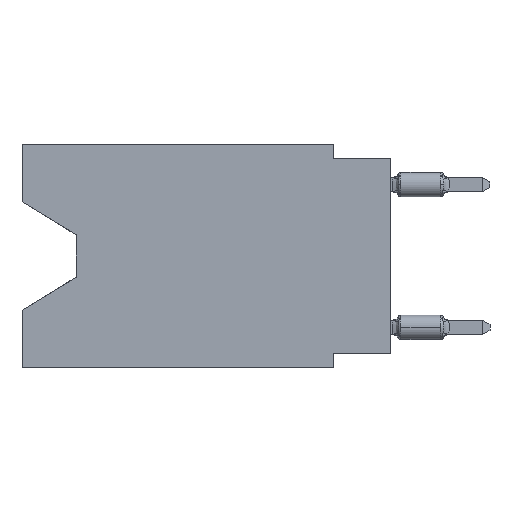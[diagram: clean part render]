
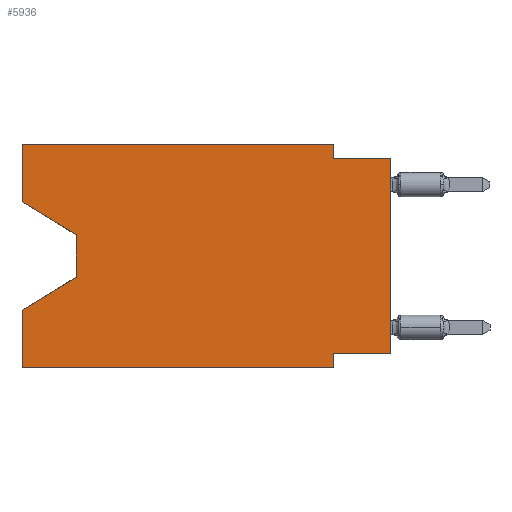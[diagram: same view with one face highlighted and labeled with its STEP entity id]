
A CAD part, left-side view. The second image highlights one B-rep face of the part: STEP entity #5936.
In plain terms, the highlighted planar face has unit normal (-1, 0, 0).
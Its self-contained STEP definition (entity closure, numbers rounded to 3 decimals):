
#179 = CARTESIAN_POINT ( 'NONE',  ( 0., 13.97, -4.013 ) ) ;
#182 = VERTEX_POINT ( 'NONE', #1026 ) ;
#193 = EDGE_CURVE ( 'NONE', #15948, #651, #8616, .T. ) ;
#277 = EDGE_CURVE ( 'NONE', #6766, #4289, #13559, .T. ) ;
#651 = VERTEX_POINT ( 'NONE', #14524 ) ;
#699 = DIRECTION ( 'NONE',  ( 0., 0., 1. ) ) ;
#1026 = CARTESIAN_POINT ( 'NONE',  ( 0., 13.97, -4.013 ) ) ;
#1091 = EDGE_CURVE ( 'NONE', #10111, #4216, #5982, .T. ) ;
#1182 = EDGE_CURVE ( 'NONE', #4814, #3480, #11240, .T. ) ;
#1298 = CARTESIAN_POINT ( 'NONE',  ( 0., 16.383, 0. ) ) ;
#1342 = EDGE_CURVE ( 'NONE', #4814, #182, #1703, .T. ) ;
#1429 = VECTOR ( 'NONE', #1827, 1000. ) ;
#1532 = VERTEX_POINT ( 'NONE', #7032 ) ;
#1703 = LINE ( 'NONE', #11560, #4851 ) ;
#1827 = DIRECTION ( 'NONE',  ( 0., -1., 0. ) ) ;
#2109 = ORIENTED_EDGE ( 'NONE', *, *, #11986, .F. ) ;
#2229 = LINE ( 'NONE', #15488, #12310 ) ;
#2294 = EDGE_CURVE ( 'NONE', #651, #9453, #3707, .T. ) ;
#2566 = ORIENTED_EDGE ( 'NONE', *, *, #15207, .F. ) ;
#2656 = LINE ( 'NONE', #12366, #3254 ) ;
#3180 = CARTESIAN_POINT ( 'NONE',  ( 0., 2.54, -9.906 ) ) ;
#3254 = VECTOR ( 'NONE', #5497, 1000. ) ;
#3269 = VECTOR ( 'NONE', #3675, 1000. ) ;
#3368 = CARTESIAN_POINT ( 'NONE',  ( 0., 0., -9.271 ) ) ;
#3475 = ORIENTED_EDGE ( 'NONE', *, *, #1182, .F. ) ;
#3480 = VERTEX_POINT ( 'NONE', #11234 ) ;
#3675 = DIRECTION ( 'NONE',  ( 0., -1., 0. ) ) ;
#3707 = LINE ( 'NONE', #13510, #9254 ) ;
#4113 = LINE ( 'NONE', #179, #4996 ) ;
#4216 = VERTEX_POINT ( 'NONE', #4569 ) ;
#4289 = VERTEX_POINT ( 'NONE', #7324 ) ;
#4407 = DIRECTION ( 'NONE',  ( 0., -1., 0. ) ) ;
#4450 = CARTESIAN_POINT ( 'NONE',  ( 0., 16.383, -9.906 ) ) ;
#4569 = CARTESIAN_POINT ( 'NONE',  ( 0., 16.383, -7.36 ) ) ;
#4804 = DIRECTION ( 'NONE',  ( 0., 0., -1. ) ) ;
#4814 = VERTEX_POINT ( 'NONE', #11020 ) ;
#4851 = VECTOR ( 'NONE', #7923, 1000. ) ;
#4869 = VECTOR ( 'NONE', #12549, 1000. ) ;
#4996 = VECTOR ( 'NONE', #9055, 1000. ) ;
#5497 = DIRECTION ( 'NONE',  ( 0., 0., 1. ) ) ;
#5936 = ADVANCED_FACE ( 'NONE', ( #15030 ), #10025, .F. ) ;
#5982 = LINE ( 'NONE', #12224, #12646 ) ;
#6018 = CARTESIAN_POINT ( 'NONE',  ( 0., 2.54, 0. ) ) ;
#6459 = ORIENTED_EDGE ( 'NONE', *, *, #1342, .T. ) ;
#6766 = VERTEX_POINT ( 'NONE', #13468 ) ;
#6854 = LINE ( 'NONE', #15508, #8143 ) ;
#7004 = ORIENTED_EDGE ( 'NONE', *, *, #11305, .T. ) ;
#7032 = CARTESIAN_POINT ( 'NONE',  ( 0., 0., -0.635 ) ) ;
#7307 = ORIENTED_EDGE ( 'NONE', *, *, #15469, .F. ) ;
#7324 = CARTESIAN_POINT ( 'NONE',  ( 0., 2.54, -0.635 ) ) ;
#7740 = CARTESIAN_POINT ( 'NONE',  ( 0., 13.97, -5.893 ) ) ;
#7923 = DIRECTION ( 'NONE',  ( 0., -0.855, -0.519 ) ) ;
#7995 = VECTOR ( 'NONE', #4804, 1000. ) ;
#8143 = VECTOR ( 'NONE', #4407, 1000. ) ;
#8616 = LINE ( 'NONE', #3368, #11880 ) ;
#8837 = AXIS2_PLACEMENT_3D ( 'NONE', #10179, #9858, #11068 ) ;
#9055 = DIRECTION ( 'NONE',  ( 0., 0., -1. ) ) ;
#9254 = VECTOR ( 'NONE', #15842, 1000. ) ;
#9453 = VERTEX_POINT ( 'NONE', #3180 ) ;
#9573 = ORIENTED_EDGE ( 'NONE', *, *, #11644, .T. ) ;
#9858 = DIRECTION ( 'NONE',  ( 1., 0., 0. ) ) ;
#10025 = PLANE ( 'NONE',  #8837 ) ;
#10029 = ORIENTED_EDGE ( 'NONE', *, *, #193, .F. ) ;
#10111 = VERTEX_POINT ( 'NONE', #7740 ) ;
#10179 = CARTESIAN_POINT ( 'NONE',  ( 0., 16.383, 0. ) ) ;
#10734 = DIRECTION ( 'NONE',  ( 0., 1., 0. ) ) ;
#10851 = DIRECTION ( 'NONE',  ( 0., 0.855, -0.519 ) ) ;
#11020 = CARTESIAN_POINT ( 'NONE',  ( 0., 16.383, -2.546 ) ) ;
#11068 = DIRECTION ( 'NONE',  ( 0., 0., -1. ) ) ;
#11080 = ORIENTED_EDGE ( 'NONE', *, *, #13390, .T. ) ;
#11234 = CARTESIAN_POINT ( 'NONE',  ( 0., 16.383, 0. ) ) ;
#11240 = LINE ( 'NONE', #1298, #4869 ) ;
#11305 = EDGE_CURVE ( 'NONE', #15948, #1532, #2656, .T. ) ;
#11560 = CARTESIAN_POINT ( 'NONE',  ( 0., 16.383, -2.546 ) ) ;
#11607 = CARTESIAN_POINT ( 'NONE',  ( 0., 16.383, 0. ) ) ;
#11644 = EDGE_CURVE ( 'NONE', #14800, #9453, #14776, .T. ) ;
#11880 = VECTOR ( 'NONE', #10734, 1000. ) ;
#11986 = EDGE_CURVE ( 'NONE', #14800, #4216, #2229, .T. ) ;
#12224 = CARTESIAN_POINT ( 'NONE',  ( 0., 13.97, -5.893 ) ) ;
#12310 = VECTOR ( 'NONE', #699, 1000. ) ;
#12366 = CARTESIAN_POINT ( 'NONE',  ( 0., 0., 0. ) ) ;
#12424 = CARTESIAN_POINT ( 'NONE',  ( 0., 16.383, -9.906 ) ) ;
#12549 = DIRECTION ( 'NONE',  ( 0., 0., 1. ) ) ;
#12646 = VECTOR ( 'NONE', #10851, 1000. ) ;
#12731 = CARTESIAN_POINT ( 'NONE',  ( 0., 0., -9.271 ) ) ;
#13075 = LINE ( 'NONE', #11607, #1429 ) ;
#13290 = ORIENTED_EDGE ( 'NONE', *, *, #1091, .T. ) ;
#13390 = EDGE_CURVE ( 'NONE', #182, #10111, #4113, .T. ) ;
#13468 = CARTESIAN_POINT ( 'NONE',  ( 0., 2.54, 0. ) ) ;
#13510 = CARTESIAN_POINT ( 'NONE',  ( 0., 2.54, -9.906 ) ) ;
#13559 = LINE ( 'NONE', #6018, #7995 ) ;
#14007 = ORIENTED_EDGE ( 'NONE', *, *, #2294, .F. ) ;
#14273 = EDGE_LOOP ( 'NONE', ( #6459, #11080, #13290, #2109, #9573, #14007, #10029, #7004, #2566, #14732, #7307, #3475 ) ) ;
#14524 = CARTESIAN_POINT ( 'NONE',  ( 0., 2.54, -9.271 ) ) ;
#14732 = ORIENTED_EDGE ( 'NONE', *, *, #277, .F. ) ;
#14776 = LINE ( 'NONE', #12424, #3269 ) ;
#14800 = VERTEX_POINT ( 'NONE', #4450 ) ;
#15030 = FACE_OUTER_BOUND ( 'NONE', #14273, .T. ) ;
#15207 = EDGE_CURVE ( 'NONE', #4289, #1532, #6854, .T. ) ;
#15469 = EDGE_CURVE ( 'NONE', #3480, #6766, #13075, .T. ) ;
#15488 = CARTESIAN_POINT ( 'NONE',  ( 0., 16.383, 0. ) ) ;
#15508 = CARTESIAN_POINT ( 'NONE',  ( 0., 0., -0.635 ) ) ;
#15842 = DIRECTION ( 'NONE',  ( 0., 0., -1. ) ) ;
#15948 = VERTEX_POINT ( 'NONE', #12731 ) ;
